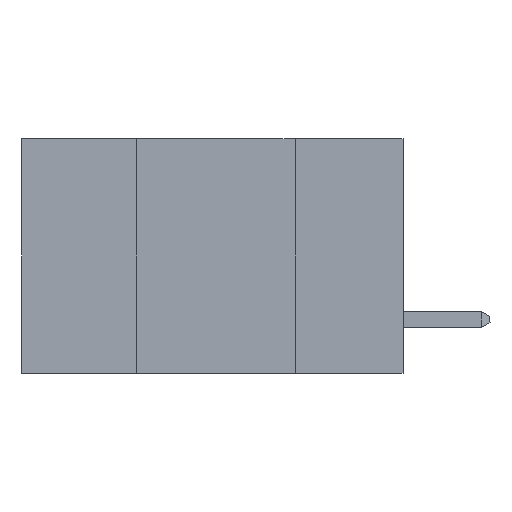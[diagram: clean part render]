
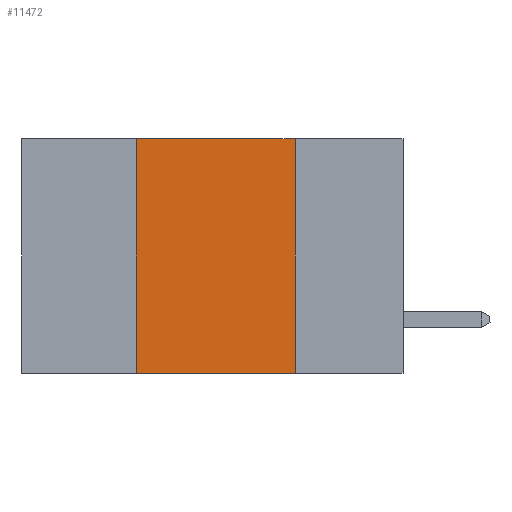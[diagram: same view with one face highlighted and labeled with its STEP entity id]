
A CAD part, left-side view. The second image highlights one B-rep face of the part: STEP entity #11472.
In plain terms, the highlighted planar face has unit normal (-1, 0, 0).
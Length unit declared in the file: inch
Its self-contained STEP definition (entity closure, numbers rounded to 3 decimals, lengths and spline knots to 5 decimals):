
#670 = ORIENTED_EDGE ( 'NONE', *, *, #10665, .F. ) ;
#685 = VERTEX_POINT ( 'NONE', #14232 ) ;
#1324 = LINE ( 'NONE', #16620, #5566 ) ;
#1605 = DIRECTION ( 'NONE',  ( 0., -1., 0. ) ) ;
#1650 = VECTOR ( 'NONE', #1605, 39.37008 ) ;
#2335 = CARTESIAN_POINT ( 'NONE',  ( 0., 0.42, 0. ) ) ;
#5071 = CARTESIAN_POINT ( 'NONE',  ( 0., 0.42, 0. ) ) ;
#5369 = VERTEX_POINT ( 'NONE', #8651 ) ;
#5566 = VECTOR ( 'NONE', #18405, 39.37008 ) ;
#5896 = CARTESIAN_POINT ( 'NONE',  ( 0., 0.42, -0.37 ) ) ;
#5914 = AXIS2_PLACEMENT_3D ( 'NONE', #6572, #20754, #10155 ) ;
#6572 = CARTESIAN_POINT ( 'NONE',  ( 0., 0.6, 0. ) ) ;
#7716 = ORIENTED_EDGE ( 'NONE', *, *, #8650, .F. ) ;
#8544 = ORIENTED_EDGE ( 'NONE', *, *, #18373, .F. ) ;
#8650 = EDGE_CURVE ( 'NONE', #16671, #19114, #11811, .T. ) ;
#8651 = CARTESIAN_POINT ( 'NONE',  ( 0., 0.17, -0.37 ) ) ;
#8689 = DIRECTION ( 'NONE',  ( 0., 0., 1. ) ) ;
#9073 = LINE ( 'NONE', #15987, #22623 ) ;
#10155 = DIRECTION ( 'NONE',  ( 0., 0., -1. ) ) ;
#10665 = EDGE_CURVE ( 'NONE', #19114, #685, #11202, .T. ) ;
#11202 = LINE ( 'NONE', #17632, #1650 ) ;
#11472 = ADVANCED_FACE ( 'NONE', ( #16991 ), #17256, .F. ) ;
#11811 = LINE ( 'NONE', #5071, #16553 ) ;
#13592 = ORIENTED_EDGE ( 'NONE', *, *, #19786, .T. ) ;
#14232 = CARTESIAN_POINT ( 'NONE',  ( 0., 0.17, 0. ) ) ;
#15501 = EDGE_LOOP ( 'NONE', ( #8544, #670, #7716, #13592 ) ) ;
#15987 = CARTESIAN_POINT ( 'NONE',  ( 0., 0.17, 0. ) ) ;
#16553 = VECTOR ( 'NONE', #8689, 39.37008 ) ;
#16620 = CARTESIAN_POINT ( 'NONE',  ( 0., 0.6, -0.37 ) ) ;
#16671 = VERTEX_POINT ( 'NONE', #5896 ) ;
#16991 = FACE_OUTER_BOUND ( 'NONE', #15501, .T. ) ;
#17256 = PLANE ( 'NONE',  #5914 ) ;
#17632 = CARTESIAN_POINT ( 'NONE',  ( 0., 0.6, 0. ) ) ;
#18373 = EDGE_CURVE ( 'NONE', #685, #5369, #9073, .T. ) ;
#18405 = DIRECTION ( 'NONE',  ( 0., -1., 0. ) ) ;
#19114 = VERTEX_POINT ( 'NONE', #2335 ) ;
#19517 = DIRECTION ( 'NONE',  ( 0., 0., -1. ) ) ;
#19786 = EDGE_CURVE ( 'NONE', #16671, #5369, #1324, .T. ) ;
#20754 = DIRECTION ( 'NONE',  ( 1., 0., 0. ) ) ;
#22623 = VECTOR ( 'NONE', #19517, 39.37008 ) ;
